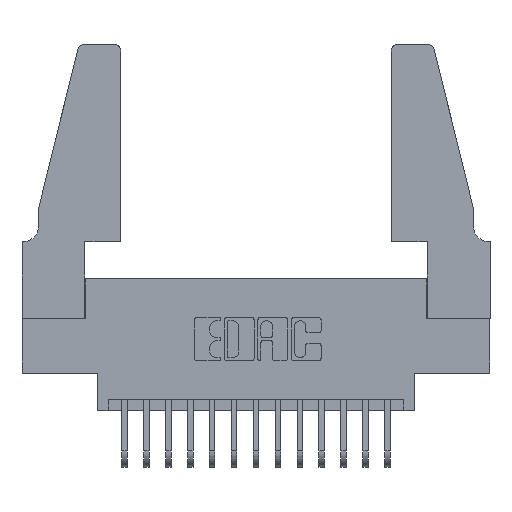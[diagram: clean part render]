
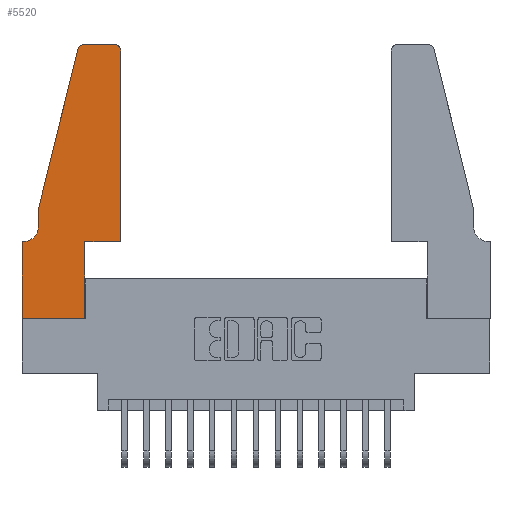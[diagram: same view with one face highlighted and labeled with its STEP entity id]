
A CAD part, top view. The second image highlights one B-rep face of the part: STEP entity #5520.
In plain terms, the highlighted planar face has unit normal (0, 0, 1).
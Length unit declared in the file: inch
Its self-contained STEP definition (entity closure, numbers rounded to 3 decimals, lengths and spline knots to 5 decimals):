
#10 = CARTESIAN_POINT ( 'NONE',  ( 0.4205, 1.25, 0.37 ) ) ;
#94 = VERTEX_POINT ( 'NONE', #3309 ) ;
#163 = VECTOR ( 'NONE', #13748, 39.37008 ) ;
#266 = ORIENTED_EDGE ( 'NONE', *, *, #13776, .T. ) ;
#323 = DIRECTION ( 'NONE',  ( -1., 0., 0. ) ) ;
#797 = CARTESIAN_POINT ( 'NONE',  ( 0., 0., 0.37 ) ) ;
#824 = AXIS2_PLACEMENT_3D ( 'NONE', #15910, #11177, #3685 ) ;
#1045 = CARTESIAN_POINT ( 'NONE',  ( 0.2865, 0.35, 0.37 ) ) ;
#1049 = AXIS2_PLACEMENT_3D ( 'NONE', #1449, #10281, #2748 ) ;
#1113 = VERTEX_POINT ( 'NONE', #12979 ) ;
#1449 = CARTESIAN_POINT ( 'NONE',  ( 0.4205, 1.22, 0.37 ) ) ;
#1591 = DIRECTION ( 'NONE',  ( 0., 0., 1. ) ) ;
#1971 = CARTESIAN_POINT ( 'NONE',  ( 0.4505, 0.35, 0.37 ) ) ;
#2288 = CARTESIAN_POINT ( 'NONE',  ( 0.0055, 0.35, 0.37 ) ) ;
#2363 = PLANE ( 'NONE',  #824 ) ;
#2748 = DIRECTION ( 'NONE',  ( 1., 0., 0. ) ) ;
#2829 = VERTEX_POINT ( 'NONE', #2288 ) ;
#3156 = AXIS2_PLACEMENT_3D ( 'NONE', #9129, #1591, #10422 ) ;
#3253 = VERTEX_POINT ( 'NONE', #8162 ) ;
#3309 = CARTESIAN_POINT ( 'NONE',  ( 0.25487, 1.22718, 0.37 ) ) ;
#3460 = EDGE_LOOP ( 'NONE', ( #6973, #9995, #14068, #266, #5347, #9099, #12307, #13256, #3750, #7015, #13601, #11027 ) ) ;
#3590 = CARTESIAN_POINT ( 'NONE',  ( 0.2865, 0.35, 0.37 ) ) ;
#3604 = VERTEX_POINT ( 'NONE', #7568 ) ;
#3619 = LINE ( 'NONE', #6285, #163 ) ;
#3685 = DIRECTION ( 'NONE',  ( 1., 0., 0. ) ) ;
#3750 = ORIENTED_EDGE ( 'NONE', *, *, #9028, .T. ) ;
#4391 = CARTESIAN_POINT ( 'NONE',  ( 0., 0.35, 0.37 ) ) ;
#4712 = VECTOR ( 'NONE', #8361, 39.37008 ) ;
#4856 = VECTOR ( 'NONE', #9888, 39.37008 ) ;
#4864 = CARTESIAN_POINT ( 'NONE',  ( 0., 0., 0.37 ) ) ;
#5347 = ORIENTED_EDGE ( 'NONE', *, *, #7995, .T. ) ;
#5470 = CARTESIAN_POINT ( 'NONE',  ( 0., 0., 0.37 ) ) ;
#5520 = ADVANCED_FACE ( 'NONE', ( #14650 ), #2363, .T. ) ;
#5869 = VERTEX_POINT ( 'NONE', #1971 ) ;
#5892 = VECTOR ( 'NONE', #7933, 39.37008 ) ;
#5955 = CIRCLE ( 'NONE', #12910, 0.07 ) ;
#6050 = EDGE_CURVE ( 'NONE', #2829, #8088, #10286, .T. ) ;
#6285 = CARTESIAN_POINT ( 'NONE',  ( 0.0755, 0.5, 0.37 ) ) ;
#6292 = DIRECTION ( 'NONE',  ( 0., -1., 0. ) ) ;
#6306 = EDGE_CURVE ( 'NONE', #1113, #7506, #16081, .T. ) ;
#6390 = VECTOR ( 'NONE', #13442, 39.37008 ) ;
#6411 = CARTESIAN_POINT ( 'NONE',  ( 0.0755, 0.42, 0.37 ) ) ;
#6804 = LINE ( 'NONE', #10030, #9724 ) ;
#6973 = ORIENTED_EDGE ( 'NONE', *, *, #15086, .T. ) ;
#7015 = ORIENTED_EDGE ( 'NONE', *, *, #14749, .T. ) ;
#7506 = VERTEX_POINT ( 'NONE', #10 ) ;
#7568 = CARTESIAN_POINT ( 'NONE',  ( 0.284, 1.25, 0.37 ) ) ;
#7908 = DIRECTION ( 'NONE',  ( 0., 0., -1. ) ) ;
#7933 = DIRECTION ( 'NONE',  ( 1., 0., 0. ) ) ;
#7995 = EDGE_CURVE ( 'NONE', #11991, #2829, #5955, .T. ) ;
#8088 = VERTEX_POINT ( 'NONE', #4391 ) ;
#8162 = CARTESIAN_POINT ( 'NONE',  ( 0.2865, 0., 0.37 ) ) ;
#8361 = DIRECTION ( 'NONE',  ( 0., -1., 0. ) ) ;
#8759 = LINE ( 'NONE', #5470, #5892 ) ;
#8771 = CIRCLE ( 'NONE', #3156, 0.03 ) ;
#9027 = VERTEX_POINT ( 'NONE', #3590 ) ;
#9028 = EDGE_CURVE ( 'NONE', #3253, #9027, #11345, .T. ) ;
#9099 = ORIENTED_EDGE ( 'NONE', *, *, #6050, .T. ) ;
#9129 = CARTESIAN_POINT ( 'NONE',  ( 0.284, 1.22, 0.37 ) ) ;
#9533 = EDGE_CURVE ( 'NONE', #8088, #13664, #13770, .T. ) ;
#9724 = VECTOR ( 'NONE', #6292, 39.37008 ) ;
#9888 = DIRECTION ( 'NONE',  ( 0., 1., 0. ) ) ;
#9995 = ORIENTED_EDGE ( 'NONE', *, *, #10943, .T. ) ;
#10020 = VERTEX_POINT ( 'NONE', #14157 ) ;
#10030 = CARTESIAN_POINT ( 'NONE',  ( 0.0755, 0.5, 0.37 ) ) ;
#10281 = DIRECTION ( 'NONE',  ( 0., 0., 1. ) ) ;
#10286 = LINE ( 'NONE', #15848, #13888 ) ;
#10422 = DIRECTION ( 'NONE',  ( 1., 0., 0. ) ) ;
#10714 = CARTESIAN_POINT ( 'NONE',  ( 0.4505, 0.35, 0.37 ) ) ;
#10943 = EDGE_CURVE ( 'NONE', #3604, #94, #8771, .T. ) ;
#11027 = ORIENTED_EDGE ( 'NONE', *, *, #6306, .T. ) ;
#11056 = DIRECTION ( 'NONE',  ( -1., 0., 0. ) ) ;
#11137 = DIRECTION ( 'NONE',  ( 0., 1., 0. ) ) ;
#11177 = DIRECTION ( 'NONE',  ( 0., 0., 1. ) ) ;
#11345 = LINE ( 'NONE', #1045, #14168 ) ;
#11462 = LINE ( 'NONE', #15897, #4856 ) ;
#11991 = VERTEX_POINT ( 'NONE', #6411 ) ;
#12207 = CARTESIAN_POINT ( 'NONE',  ( 0.2605, 1.25, 0.37 ) ) ;
#12307 = ORIENTED_EDGE ( 'NONE', *, *, #9533, .T. ) ;
#12910 = AXIS2_PLACEMENT_3D ( 'NONE', #15227, #7908, #323 ) ;
#12979 = CARTESIAN_POINT ( 'NONE',  ( 0.4505, 1.22, 0.37 ) ) ;
#13224 = EDGE_CURVE ( 'NONE', #13664, #3253, #8759, .T. ) ;
#13256 = ORIENTED_EDGE ( 'NONE', *, *, #13224, .T. ) ;
#13442 = DIRECTION ( 'NONE',  ( -1., 0., 0. ) ) ;
#13601 = ORIENTED_EDGE ( 'NONE', *, *, #14330, .T. ) ;
#13664 = VERTEX_POINT ( 'NONE', #4864 ) ;
#13748 = DIRECTION ( 'NONE',  ( -0.239, -0.971, 0. ) ) ;
#13770 = LINE ( 'NONE', #797, #4712 ) ;
#13776 = EDGE_CURVE ( 'NONE', #10020, #11991, #6804, .T. ) ;
#13888 = VECTOR ( 'NONE', #11056, 39.37008 ) ;
#14068 = ORIENTED_EDGE ( 'NONE', *, *, #15238, .T. ) ;
#14157 = CARTESIAN_POINT ( 'NONE',  ( 0.0755, 0.5, 0.37 ) ) ;
#14168 = VECTOR ( 'NONE', #11137, 39.37008 ) ;
#14272 = VECTOR ( 'NONE', #15515, 39.37008 ) ;
#14330 = EDGE_CURVE ( 'NONE', #5869, #1113, #11462, .T. ) ;
#14641 = LINE ( 'NONE', #10714, #14272 ) ;
#14650 = FACE_OUTER_BOUND ( 'NONE', #3460, .T. ) ;
#14749 = EDGE_CURVE ( 'NONE', #9027, #5869, #14641, .T. ) ;
#15086 = EDGE_CURVE ( 'NONE', #7506, #3604, #15587, .T. ) ;
#15227 = CARTESIAN_POINT ( 'NONE',  ( 0.0055, 0.42, 0.37 ) ) ;
#15238 = EDGE_CURVE ( 'NONE', #94, #10020, #3619, .T. ) ;
#15515 = DIRECTION ( 'NONE',  ( 1., 0., 0. ) ) ;
#15587 = LINE ( 'NONE', #12207, #6390 ) ;
#15848 = CARTESIAN_POINT ( 'NONE',  ( 0.0755, 0.35, 0.37 ) ) ;
#15897 = CARTESIAN_POINT ( 'NONE',  ( 0.4505, 0.35, 0.37 ) ) ;
#15910 = CARTESIAN_POINT ( 'NONE',  ( 0., 0.35, 0.37 ) ) ;
#16081 = CIRCLE ( 'NONE', #1049, 0.03 ) ;
